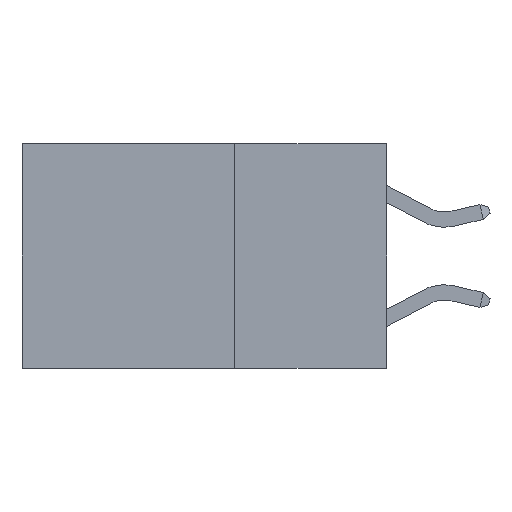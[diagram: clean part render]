
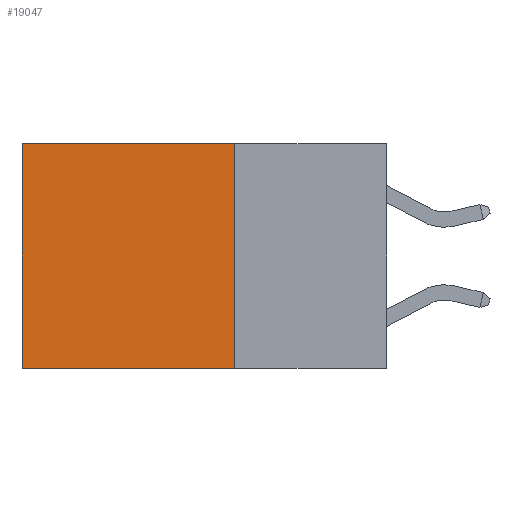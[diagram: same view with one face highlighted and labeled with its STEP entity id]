
A CAD part, left-side view. The second image highlights one B-rep face of the part: STEP entity #19047.
In plain terms, the highlighted planar face has unit normal (-1, 0, 0).
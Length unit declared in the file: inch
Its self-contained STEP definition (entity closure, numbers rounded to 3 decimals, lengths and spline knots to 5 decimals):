
#933 = CARTESIAN_POINT ( 'NONE',  ( 0.2625, 0.6, -0.37 ) ) ;
#1067 = ORIENTED_EDGE ( 'NONE', *, *, #18335, .T. ) ;
#1389 = VERTEX_POINT ( 'NONE', #12704 ) ;
#2054 = DIRECTION ( 'NONE',  ( 0., 0., -1. ) ) ;
#2274 = VECTOR ( 'NONE', #7813, 39.37008 ) ;
#2936 = AXIS2_PLACEMENT_3D ( 'NONE', #8551, #7091, #4240 ) ;
#3053 = VECTOR ( 'NONE', #2054, 39.37008 ) ;
#4049 = VERTEX_POINT ( 'NONE', #933 ) ;
#4240 = DIRECTION ( 'NONE',  ( 0., 0., -1. ) ) ;
#4831 = EDGE_CURVE ( 'NONE', #1389, #10484, #15450, .T. ) ;
#5026 = LINE ( 'NONE', #17257, #5876 ) ;
#5876 = VECTOR ( 'NONE', #17164, 39.37008 ) ;
#6161 = CARTESIAN_POINT ( 'NONE',  ( 0.2625, 0.6, 0. ) ) ;
#6550 = ORIENTED_EDGE ( 'NONE', *, *, #9598, .T. ) ;
#6653 = EDGE_LOOP ( 'NONE', ( #1067, #13748, #13408, #6550 ) ) ;
#6865 = CARTESIAN_POINT ( 'NONE',  ( 0.2625, 0.6, 0. ) ) ;
#7048 = CARTESIAN_POINT ( 'NONE',  ( 0.2625, 0.25, -0.37 ) ) ;
#7091 = DIRECTION ( 'NONE',  ( 1., 0., 0. ) ) ;
#7813 = DIRECTION ( 'NONE',  ( 0., 0., -1. ) ) ;
#8551 = CARTESIAN_POINT ( 'NONE',  ( 0.2625, 0.25, 0. ) ) ;
#9598 = EDGE_CURVE ( 'NONE', #1389, #12484, #5026, .T. ) ;
#10484 = VERTEX_POINT ( 'NONE', #11041 ) ;
#11041 = CARTESIAN_POINT ( 'NONE',  ( 0.2625, 0.25, -0.37 ) ) ;
#11377 = EDGE_CURVE ( 'NONE', #10484, #4049, #16051, .T. ) ;
#12484 = VERTEX_POINT ( 'NONE', #6865 ) ;
#12704 = CARTESIAN_POINT ( 'NONE',  ( 0.2625, 0.25, 0. ) ) ;
#13408 = ORIENTED_EDGE ( 'NONE', *, *, #4831, .F. ) ;
#13438 = VECTOR ( 'NONE', #17425, 39.37008 ) ;
#13748 = ORIENTED_EDGE ( 'NONE', *, *, #11377, .F. ) ;
#14078 = CARTESIAN_POINT ( 'NONE',  ( 0.2625, 0.25, 0. ) ) ;
#15450 = LINE ( 'NONE', #14078, #3053 ) ;
#16051 = LINE ( 'NONE', #7048, #13438 ) ;
#16621 = LINE ( 'NONE', #6161, #2274 ) ;
#17164 = DIRECTION ( 'NONE',  ( 0., 1., 0. ) ) ;
#17257 = CARTESIAN_POINT ( 'NONE',  ( 0.2625, 0.25, 0. ) ) ;
#17425 = DIRECTION ( 'NONE',  ( 0., 1., 0. ) ) ;
#18335 = EDGE_CURVE ( 'NONE', #12484, #4049, #16621, .T. ) ;
#19047 = ADVANCED_FACE ( 'NONE', ( #19105 ), #19206, .F. ) ;
#19105 = FACE_OUTER_BOUND ( 'NONE', #6653, .T. ) ;
#19206 = PLANE ( 'NONE',  #2936 ) ;
